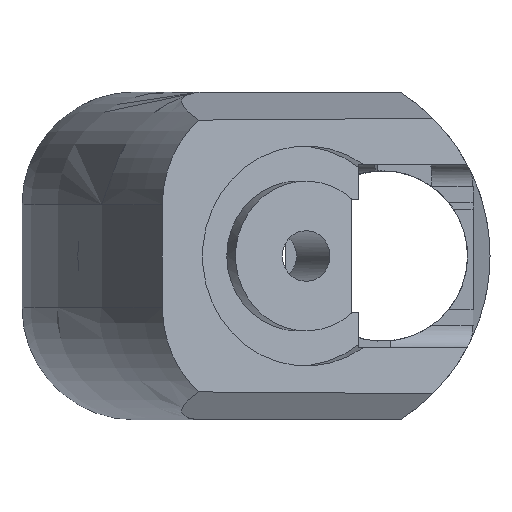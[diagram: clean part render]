
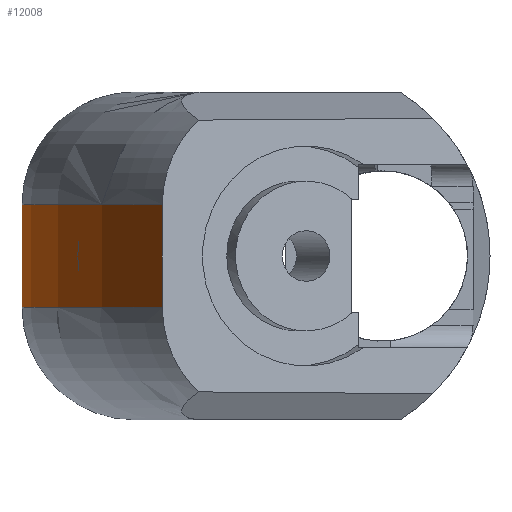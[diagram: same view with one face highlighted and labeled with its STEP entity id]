
A CAD part, left-side view. The second image highlights one B-rep face of the part: STEP entity #12008.
In plain terms, the highlighted cylindrical face has radius 197.297 mm (diameter 394.594 mm), a partial arc.
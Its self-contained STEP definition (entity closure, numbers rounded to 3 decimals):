
#157 = TOROIDAL_SURFACE('',#158,182.057,15.24);
#158 = AXIS2_PLACEMENT_3D('',#159,#160,#161);
#159 = CARTESIAN_POINT('',(-124.968,-133.797,-6.985));
#160 = DIRECTION('',(0.,0.,1.));
#161 = DIRECTION('',(0.,1.,0.));
#1723 = PLANE('',#1724);
#1724 = AXIS2_PLACEMENT_3D('',#1725,#1726,#1727);
#1725 = CARTESIAN_POINT('',(-209.55,44.45,-22.225));
#1726 = DIRECTION('',(0.943,0.334,0.));
#1727 = DIRECTION('',(0.334,-0.943,0.));
#1896 = PLANE('',#1897);
#1897 = AXIS2_PLACEMENT_3D('',#1898,#1899,#1900);
#1898 = CARTESIAN_POINT('',(0.,63.5,-22.225));
#1899 = DIRECTION('',(0.,-1.,0.));
#1900 = DIRECTION('',(-1.,0.,0.));
#3564 = VERTEX_POINT('',#3565);
#3565 = CARTESIAN_POINT('',(-124.968,63.5,-6.985));
#3613 = VERTEX_POINT('',#3614);
#3614 = CARTESIAN_POINT('',(-209.55,44.45,-6.985));
#3772 = EDGE_CURVE('',#3564,#3613,#3773,.T.);
#3773 = SURFACE_CURVE('',#3774,(#3779,#3786),.PCURVE_S1.);
#3774 = CIRCLE('',#3775,197.297);
#3775 = AXIS2_PLACEMENT_3D('',#3776,#3777,#3778);
#3776 = CARTESIAN_POINT('',(-124.968,-133.797,-6.985));
#3777 = DIRECTION('',(0.,0.,1.));
#3778 = DIRECTION('',(0.,1.,0.));
#3779 = PCURVE('',#157,#3780);
#3780 = DEFINITIONAL_REPRESENTATION('',(#3781),#3785);
#3781 = LINE('',#3782,#3783);
#3782 = CARTESIAN_POINT('',(0.,6.283));
#3783 = VECTOR('',#3784,1.);
#3784 = DIRECTION('',(1.,0.));
#3785 = ( GEOMETRIC_REPRESENTATION_CONTEXT(2) 
PARAMETRIC_REPRESENTATION_CONTEXT() REPRESENTATION_CONTEXT('2D SPACE',''
  ) );
#3786 = PCURVE('',#3787,#3792);
#3787 = CYLINDRICAL_SURFACE('',#3788,197.297);
#3788 = AXIS2_PLACEMENT_3D('',#3789,#3790,#3791);
#3789 = CARTESIAN_POINT('',(-124.968,-133.797,-22.225));
#3790 = DIRECTION('',(0.,0.,-1.));
#3791 = DIRECTION('',(1.,0.,0.));
#3792 = DEFINITIONAL_REPRESENTATION('',(#3793),#3797);
#3793 = LINE('',#3794,#3795);
#3794 = CARTESIAN_POINT('',(-1.571,-15.24));
#3795 = VECTOR('',#3796,1.);
#3796 = DIRECTION('',(-1.,0.));
#3797 = ( GEOMETRIC_REPRESENTATION_CONTEXT(2) 
PARAMETRIC_REPRESENTATION_CONTEXT() REPRESENTATION_CONTEXT('2D SPACE',''
  ) );
#4520 = EDGE_CURVE('',#3613,#4521,#4523,.T.);
#4521 = VERTEX_POINT('',#4522);
#4522 = CARTESIAN_POINT('',(-209.55,44.45,6.985));
#4523 = SURFACE_CURVE('',#4524,(#4528,#4535),.PCURVE_S1.);
#4524 = LINE('',#4525,#4526);
#4525 = CARTESIAN_POINT('',(-209.55,44.45,-22.225));
#4526 = VECTOR('',#4527,1.);
#4527 = DIRECTION('',(0.,0.,1.));
#4528 = PCURVE('',#1723,#4529);
#4529 = DEFINITIONAL_REPRESENTATION('',(#4530),#4534);
#4530 = LINE('',#4531,#4532);
#4531 = CARTESIAN_POINT('',(0.,-0.));
#4532 = VECTOR('',#4533,1.);
#4533 = DIRECTION('',(0.,-1.));
#4534 = ( GEOMETRIC_REPRESENTATION_CONTEXT(2) 
PARAMETRIC_REPRESENTATION_CONTEXT() REPRESENTATION_CONTEXT('2D SPACE',''
  ) );
#4535 = PCURVE('',#3787,#4536);
#4536 = DEFINITIONAL_REPRESENTATION('',(#4537),#4541);
#4537 = LINE('',#4538,#4539);
#4538 = CARTESIAN_POINT('',(-2.014,0.));
#4539 = VECTOR('',#4540,1.);
#4540 = DIRECTION('',(-0.,-1.));
#4541 = ( GEOMETRIC_REPRESENTATION_CONTEXT(2) 
PARAMETRIC_REPRESENTATION_CONTEXT() REPRESENTATION_CONTEXT('2D SPACE',''
  ) );
#4597 = TOROIDAL_SURFACE('',#4598,182.057,15.24);
#4598 = AXIS2_PLACEMENT_3D('',#4599,#4600,#4601);
#4599 = CARTESIAN_POINT('',(-124.968,-133.797,6.985));
#4600 = DIRECTION('',(0.,0.,-1.));
#4601 = DIRECTION('',(0.,1.,0.));
#7270 = VERTEX_POINT('',#7271);
#7271 = CARTESIAN_POINT('',(-124.968,63.5,6.985));
#7543 = EDGE_CURVE('',#3564,#7270,#7544,.T.);
#7544 = SURFACE_CURVE('',#7545,(#7549,#7556),.PCURVE_S1.);
#7545 = LINE('',#7546,#7547);
#7546 = CARTESIAN_POINT('',(-124.968,63.5,-22.225));
#7547 = VECTOR('',#7548,1.);
#7548 = DIRECTION('',(0.,0.,1.));
#7549 = PCURVE('',#1896,#7550);
#7550 = DEFINITIONAL_REPRESENTATION('',(#7551),#7555);
#7551 = LINE('',#7552,#7553);
#7552 = CARTESIAN_POINT('',(124.968,0.));
#7553 = VECTOR('',#7554,1.);
#7554 = DIRECTION('',(0.,-1.));
#7555 = ( GEOMETRIC_REPRESENTATION_CONTEXT(2) 
PARAMETRIC_REPRESENTATION_CONTEXT() REPRESENTATION_CONTEXT('2D SPACE',''
  ) );
#7556 = PCURVE('',#3787,#7557);
#7557 = DEFINITIONAL_REPRESENTATION('',(#7558),#7562);
#7558 = LINE('',#7559,#7560);
#7559 = CARTESIAN_POINT('',(-1.571,0.));
#7560 = VECTOR('',#7561,1.);
#7561 = DIRECTION('',(-0.,-1.));
#7562 = ( GEOMETRIC_REPRESENTATION_CONTEXT(2) 
PARAMETRIC_REPRESENTATION_CONTEXT() REPRESENTATION_CONTEXT('2D SPACE',''
  ) );
#12008 = ADVANCED_FACE('',(#12009),#3787,.T.);
#12009 = FACE_BOUND('',#12010,.F.);
#12010 = EDGE_LOOP('',(#12011,#12012,#12034,#12035));
#12011 = ORIENTED_EDGE('',*,*,#7543,.T.);
#12012 = ORIENTED_EDGE('',*,*,#12013,.T.);
#12013 = EDGE_CURVE('',#7270,#4521,#12014,.T.);
#12014 = SURFACE_CURVE('',#12015,(#12020,#12027),.PCURVE_S1.);
#12015 = CIRCLE('',#12016,197.297);
#12016 = AXIS2_PLACEMENT_3D('',#12017,#12018,#12019);
#12017 = CARTESIAN_POINT('',(-124.968,-133.797,6.985));
#12018 = DIRECTION('',(0.,0.,1.));
#12019 = DIRECTION('',(0.,1.,0.));
#12020 = PCURVE('',#3787,#12021);
#12021 = DEFINITIONAL_REPRESENTATION('',(#12022),#12026);
#12022 = LINE('',#12023,#12024);
#12023 = CARTESIAN_POINT('',(-1.571,-29.21));
#12024 = VECTOR('',#12025,1.);
#12025 = DIRECTION('',(-1.,0.));
#12026 = ( GEOMETRIC_REPRESENTATION_CONTEXT(2) 
PARAMETRIC_REPRESENTATION_CONTEXT() REPRESENTATION_CONTEXT('2D SPACE',''
  ) );
#12027 = PCURVE('',#4597,#12028);
#12028 = DEFINITIONAL_REPRESENTATION('',(#12029),#12033);
#12029 = LINE('',#12030,#12031);
#12030 = CARTESIAN_POINT('',(-0.,6.283));
#12031 = VECTOR('',#12032,1.);
#12032 = DIRECTION('',(-1.,0.));
#12033 = ( GEOMETRIC_REPRESENTATION_CONTEXT(2) 
PARAMETRIC_REPRESENTATION_CONTEXT() REPRESENTATION_CONTEXT('2D SPACE',''
  ) );
#12034 = ORIENTED_EDGE('',*,*,#4520,.F.);
#12035 = ORIENTED_EDGE('',*,*,#3772,.F.);
